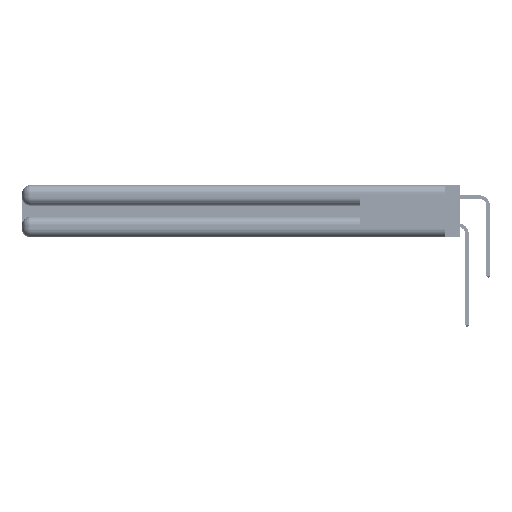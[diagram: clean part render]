
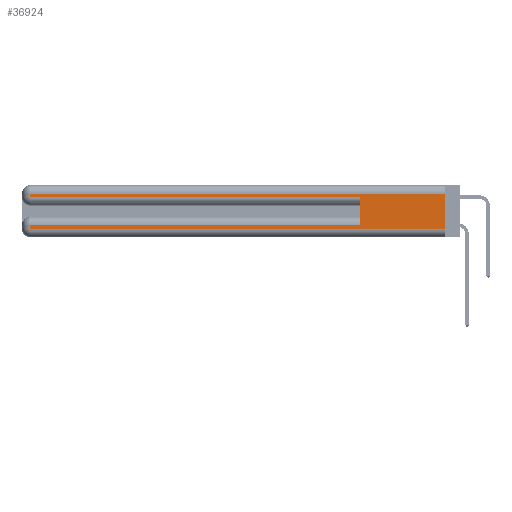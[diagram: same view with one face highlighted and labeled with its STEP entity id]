
A CAD part, left-side view. The second image highlights one B-rep face of the part: STEP entity #36924.
In plain terms, the highlighted planar face has unit normal (-1, 0, 0).
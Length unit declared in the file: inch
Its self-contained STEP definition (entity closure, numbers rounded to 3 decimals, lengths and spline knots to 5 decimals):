
#233 = ORIENTED_EDGE ( 'NONE', *, *, #13287, .T. ) ;
#794 = LINE ( 'NONE', #24333, #21398 ) ;
#936 = LINE ( 'NONE', #18093, #16716 ) ;
#1126 = CARTESIAN_POINT ( 'NONE',  ( 0., 0.6, 0.145 ) ) ;
#6100 = VERTEX_POINT ( 'NONE', #43915 ) ;
#6278 = LINE ( 'NONE', #1126, #44095 ) ;
#6298 = ORIENTED_EDGE ( 'NONE', *, *, #7239, .T. ) ;
#6748 = VERTEX_POINT ( 'NONE', #23108 ) ;
#6872 = DIRECTION ( 'NONE',  ( 0., -1., 0. ) ) ;
#7097 = LINE ( 'NONE', #18655, #46264 ) ;
#7239 = EDGE_CURVE ( 'NONE', #21209, #30996, #25508, .T. ) ;
#7490 = ORIENTED_EDGE ( 'NONE', *, *, #31984, .T. ) ;
#8154 = CARTESIAN_POINT ( 'NONE',  ( 0., 2.94, 0.31 ) ) ;
#8787 = EDGE_CURVE ( 'NONE', #54018, #21209, #14960, .T. ) ;
#10224 = CARTESIAN_POINT ( 'NONE',  ( 0., 2.94, 0.085 ) ) ;
#10932 = CARTESIAN_POINT ( 'NONE',  ( 0., 0., 0.06 ) ) ;
#11597 = CARTESIAN_POINT ( 'NONE',  ( 0., 2.94, 0.285 ) ) ;
#13287 = EDGE_CURVE ( 'NONE', #30996, #22549, #35796, .T. ) ;
#13440 = AXIS2_PLACEMENT_3D ( 'NONE', #30698, #39545, #35335 ) ;
#14100 = ORIENTED_EDGE ( 'NONE', *, *, #15703, .F. ) ;
#14630 = DIRECTION ( 'NONE',  ( 0., 1., 0. ) ) ;
#14892 = CARTESIAN_POINT ( 'NONE',  ( 0., 0., 0.085 ) ) ;
#14960 = LINE ( 'NONE', #14892, #30018 ) ;
#15703 = EDGE_CURVE ( 'NONE', #54018, #6100, #6278, .T. ) ;
#16716 = VECTOR ( 'NONE', #53217, 39.37008 ) ;
#17539 = EDGE_LOOP ( 'NONE', ( #50448, #47647, #7490, #52536, #14100, #51749, #6298, #233 ) ) ;
#17715 = CARTESIAN_POINT ( 'NONE',  ( 0., 2.94, 0.37 ) ) ;
#18093 = CARTESIAN_POINT ( 'NONE',  ( 0., 0., 0.37 ) ) ;
#18655 = CARTESIAN_POINT ( 'NONE',  ( 0., 0., 0.31 ) ) ;
#20950 = EDGE_CURVE ( 'NONE', #51077, #6100, #794, .T. ) ;
#21209 = VERTEX_POINT ( 'NONE', #10224 ) ;
#21398 = VECTOR ( 'NONE', #6872, 39.37008 ) ;
#22549 = VERTEX_POINT ( 'NONE', #10932 ) ;
#23108 = CARTESIAN_POINT ( 'NONE',  ( 0., 0., 0.31 ) ) ;
#23190 = DIRECTION ( 'NONE',  ( 0., 0., 1. ) ) ;
#24333 = CARTESIAN_POINT ( 'NONE',  ( 0., 0., 0.285 ) ) ;
#25410 = LINE ( 'NONE', #50180, #38541 ) ;
#25508 = LINE ( 'NONE', #17715, #31136 ) ;
#30018 = VECTOR ( 'NONE', #45757, 39.37008 ) ;
#30698 = CARTESIAN_POINT ( 'NONE',  ( 0., 0., 0.37 ) ) ;
#30996 = VERTEX_POINT ( 'NONE', #42612 ) ;
#31136 = VECTOR ( 'NONE', #39955, 39.37008 ) ;
#31381 = CARTESIAN_POINT ( 'NONE',  ( 0., 0.6, 0.085 ) ) ;
#31984 = EDGE_CURVE ( 'NONE', #55555, #51077, #25410, .T. ) ;
#34051 = DIRECTION ( 'NONE',  ( 0., -1., 0. ) ) ;
#35335 = DIRECTION ( 'NONE',  ( 0., 0., -1. ) ) ;
#35796 = LINE ( 'NONE', #51294, #48815 ) ;
#36924 = ADVANCED_FACE ( 'NONE', ( #50013 ), #39371, .F. ) ;
#38541 = VECTOR ( 'NONE', #46148, 39.37008 ) ;
#39371 = PLANE ( 'NONE',  #13440 ) ;
#39545 = DIRECTION ( 'NONE',  ( 1., 0., 0. ) ) ;
#39955 = DIRECTION ( 'NONE',  ( 0., 0., -1. ) ) ;
#42612 = CARTESIAN_POINT ( 'NONE',  ( 0., 2.94, 0.06 ) ) ;
#43915 = CARTESIAN_POINT ( 'NONE',  ( 0., 0.6, 0.285 ) ) ;
#44095 = VECTOR ( 'NONE', #23190, 39.37008 ) ;
#45757 = DIRECTION ( 'NONE',  ( 0., 1., 0. ) ) ;
#46148 = DIRECTION ( 'NONE',  ( 0., 0., -1. ) ) ;
#46264 = VECTOR ( 'NONE', #14630, 39.37008 ) ;
#47647 = ORIENTED_EDGE ( 'NONE', *, *, #47785, .T. ) ;
#47785 = EDGE_CURVE ( 'NONE', #6748, #55555, #7097, .T. ) ;
#48815 = VECTOR ( 'NONE', #34051, 39.37008 ) ;
#50013 = FACE_OUTER_BOUND ( 'NONE', #17539, .T. ) ;
#50180 = CARTESIAN_POINT ( 'NONE',  ( 0., 2.94, 0.37 ) ) ;
#50448 = ORIENTED_EDGE ( 'NONE', *, *, #52790, .F. ) ;
#51077 = VERTEX_POINT ( 'NONE', #11597 ) ;
#51294 = CARTESIAN_POINT ( 'NONE',  ( 0., 0., 0.06 ) ) ;
#51749 = ORIENTED_EDGE ( 'NONE', *, *, #8787, .T. ) ;
#52536 = ORIENTED_EDGE ( 'NONE', *, *, #20950, .T. ) ;
#52790 = EDGE_CURVE ( 'NONE', #6748, #22549, #936, .T. ) ;
#53217 = DIRECTION ( 'NONE',  ( 0., 0., -1. ) ) ;
#54018 = VERTEX_POINT ( 'NONE', #31381 ) ;
#55555 = VERTEX_POINT ( 'NONE', #8154 ) ;
